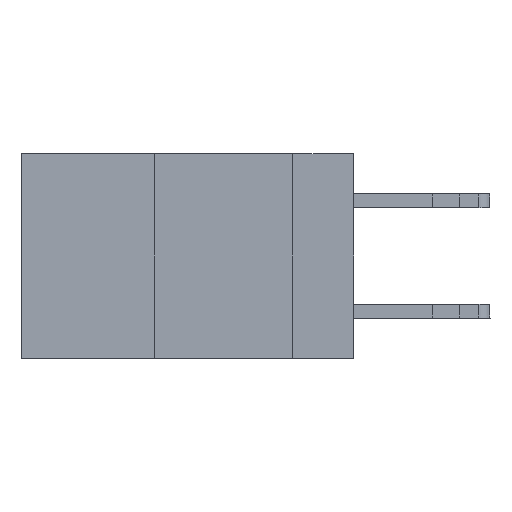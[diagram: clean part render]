
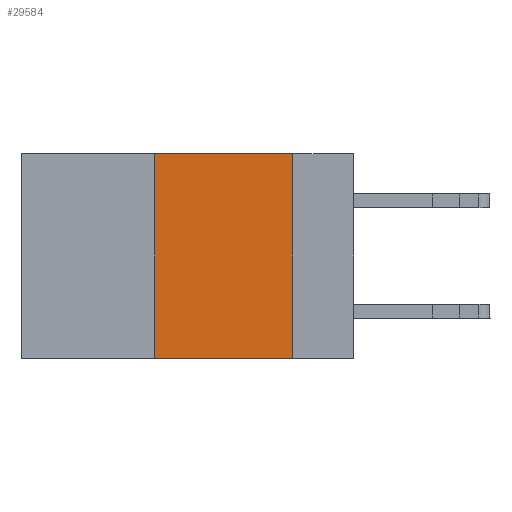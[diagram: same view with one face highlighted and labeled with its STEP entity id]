
A CAD part, left-side view. The second image highlights one B-rep face of the part: STEP entity #29584.
In plain terms, the highlighted planar face has unit normal (-1, 0, 0).
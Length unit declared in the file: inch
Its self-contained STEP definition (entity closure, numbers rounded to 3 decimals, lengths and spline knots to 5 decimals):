
#1470 = LINE ( 'NONE', #22331, #25930 ) ;
#2130 = EDGE_CURVE ( 'NONE', #28605, #29263, #1470, .T. ) ;
#3976 = EDGE_CURVE ( 'NONE', #16127, #29263, #31664, .T. ) ;
#4144 = PLANE ( 'NONE',  #4538 ) ;
#4275 = VECTOR ( 'NONE', #20529, 39.37008 ) ;
#4538 = AXIS2_PLACEMENT_3D ( 'NONE', #31143, #18889, #23910 ) ;
#5417 = DIRECTION ( 'NONE',  ( 0., 0., -1. ) ) ;
#5778 = CARTESIAN_POINT ( 'NONE',  ( 0., 0.36, 0. ) ) ;
#6650 = EDGE_CURVE ( 'NONE', #23585, #28605, #29990, .T. ) ;
#7813 = FACE_OUTER_BOUND ( 'NONE', #28713, .T. ) ;
#10757 = ORIENTED_EDGE ( 'NONE', *, *, #6650, .F. ) ;
#11914 = LINE ( 'NONE', #20751, #4275 ) ;
#16127 = VERTEX_POINT ( 'NONE', #25988 ) ;
#16498 = DIRECTION ( 'NONE',  ( 0., -1., 0. ) ) ;
#17491 = ORIENTED_EDGE ( 'NONE', *, *, #23565, .F. ) ;
#18889 = DIRECTION ( 'NONE',  ( 1., 0., 0. ) ) ;
#20433 = ORIENTED_EDGE ( 'NONE', *, *, #2130, .F. ) ;
#20529 = DIRECTION ( 'NONE',  ( 0., 0., 1. ) ) ;
#20751 = CARTESIAN_POINT ( 'NONE',  ( 0., 0.36, 0. ) ) ;
#21509 = CARTESIAN_POINT ( 'NONE',  ( 0., 0.6, 0. ) ) ;
#22124 = DIRECTION ( 'NONE',  ( 0., -1., 0. ) ) ;
#22331 = CARTESIAN_POINT ( 'NONE',  ( 0., 0.11, 0. ) ) ;
#23565 = EDGE_CURVE ( 'NONE', #16127, #23585, #11914, .T. ) ;
#23585 = VERTEX_POINT ( 'NONE', #5778 ) ;
#23910 = DIRECTION ( 'NONE',  ( 0., 0., -1. ) ) ;
#25879 = CARTESIAN_POINT ( 'NONE',  ( 0., 0.6, -0.37 ) ) ;
#25930 = VECTOR ( 'NONE', #5417, 39.37008 ) ;
#25988 = CARTESIAN_POINT ( 'NONE',  ( 0., 0.36, -0.37 ) ) ;
#26185 = ORIENTED_EDGE ( 'NONE', *, *, #3976, .T. ) ;
#26875 = CARTESIAN_POINT ( 'NONE',  ( 0., 0.11, -0.37 ) ) ;
#27390 = VECTOR ( 'NONE', #22124, 39.37008 ) ;
#28605 = VERTEX_POINT ( 'NONE', #29050 ) ;
#28713 = EDGE_LOOP ( 'NONE', ( #20433, #10757, #17491, #26185 ) ) ;
#29050 = CARTESIAN_POINT ( 'NONE',  ( 0., 0.11, 0. ) ) ;
#29220 = VECTOR ( 'NONE', #16498, 39.37008 ) ;
#29263 = VERTEX_POINT ( 'NONE', #26875 ) ;
#29584 = ADVANCED_FACE ( 'NONE', ( #7813 ), #4144, .F. ) ;
#29990 = LINE ( 'NONE', #21509, #29220 ) ;
#31143 = CARTESIAN_POINT ( 'NONE',  ( 0., 0.6, 0. ) ) ;
#31664 = LINE ( 'NONE', #25879, #27390 ) ;
